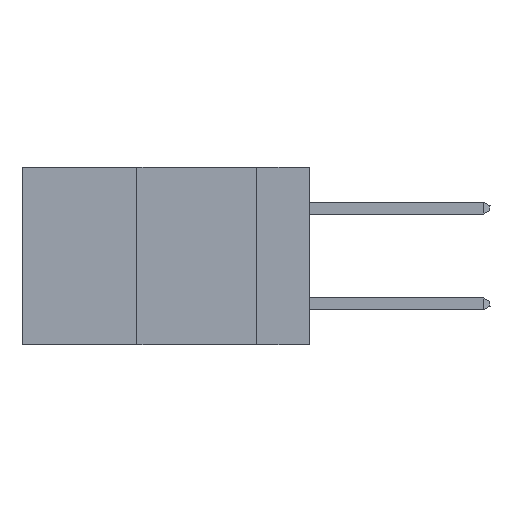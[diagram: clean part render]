
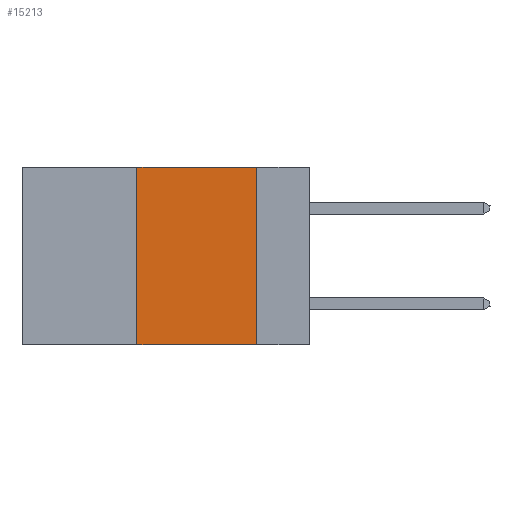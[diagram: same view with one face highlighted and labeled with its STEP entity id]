
A CAD part, left-side view. The second image highlights one B-rep face of the part: STEP entity #15213.
In plain terms, the highlighted planar face has unit normal (-1, 0, 0).
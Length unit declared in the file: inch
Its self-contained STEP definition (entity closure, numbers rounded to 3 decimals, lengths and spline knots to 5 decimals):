
#1571 = FACE_OUTER_BOUND ( 'NONE', #30304, .T. ) ;
#1800 = CARTESIAN_POINT ( 'NONE',  ( 0., 0.6, 0. ) ) ;
#1911 = DIRECTION ( 'NONE',  ( 1., 0., 0. ) ) ;
#2174 = VECTOR ( 'NONE', #3909, 39.37008 ) ;
#2556 = VECTOR ( 'NONE', #25964, 39.37008 ) ;
#3476 = EDGE_CURVE ( 'NONE', #14570, #18994, #7457, .T. ) ;
#3909 = DIRECTION ( 'NONE',  ( 0., 0., -1. ) ) ;
#4589 = EDGE_CURVE ( 'NONE', #14570, #4740, #16240, .T. ) ;
#4740 = VERTEX_POINT ( 'NONE', #10432 ) ;
#5135 = DIRECTION ( 'NONE',  ( 0., -1., 0. ) ) ;
#5413 = LINE ( 'NONE', #17313, #27243 ) ;
#5538 = VECTOR ( 'NONE', #17317, 39.37008 ) ;
#7457 = LINE ( 'NONE', #13384, #2556 ) ;
#9058 = VERTEX_POINT ( 'NONE', #29361 ) ;
#9211 = AXIS2_PLACEMENT_3D ( 'NONE', #1800, #1911, #11450 ) ;
#10432 = CARTESIAN_POINT ( 'NONE',  ( 0., 0.11, -0.37 ) ) ;
#11450 = DIRECTION ( 'NONE',  ( 0., 0., -1. ) ) ;
#13384 = CARTESIAN_POINT ( 'NONE',  ( 0., 0.36, 0. ) ) ;
#14570 = VERTEX_POINT ( 'NONE', #27188 ) ;
#15213 = ADVANCED_FACE ( 'NONE', ( #1571 ), #26151, .F. ) ;
#15814 = ORIENTED_EDGE ( 'NONE', *, *, #21680, .F. ) ;
#16240 = LINE ( 'NONE', #24626, #5538 ) ;
#17313 = CARTESIAN_POINT ( 'NONE',  ( 0., 0.6, 0. ) ) ;
#17317 = DIRECTION ( 'NONE',  ( 0., -1., 0. ) ) ;
#18544 = CARTESIAN_POINT ( 'NONE',  ( 0., 0.11, 0. ) ) ;
#18994 = VERTEX_POINT ( 'NONE', #26664 ) ;
#19139 = ORIENTED_EDGE ( 'NONE', *, *, #3476, .F. ) ;
#21283 = LINE ( 'NONE', #18544, #2174 ) ;
#21680 = EDGE_CURVE ( 'NONE', #9058, #4740, #21283, .T. ) ;
#24626 = CARTESIAN_POINT ( 'NONE',  ( 0., 0.6, -0.37 ) ) ;
#25964 = DIRECTION ( 'NONE',  ( 0., 0., 1. ) ) ;
#26151 = PLANE ( 'NONE',  #9211 ) ;
#26664 = CARTESIAN_POINT ( 'NONE',  ( 0., 0.36, 0. ) ) ;
#27188 = CARTESIAN_POINT ( 'NONE',  ( 0., 0.36, -0.37 ) ) ;
#27243 = VECTOR ( 'NONE', #5135, 39.37008 ) ;
#29361 = CARTESIAN_POINT ( 'NONE',  ( 0., 0.11, 0. ) ) ;
#30304 = EDGE_LOOP ( 'NONE', ( #15814, #30993, #19139, #30521 ) ) ;
#30521 = ORIENTED_EDGE ( 'NONE', *, *, #4589, .T. ) ;
#30713 = EDGE_CURVE ( 'NONE', #18994, #9058, #5413, .T. ) ;
#30993 = ORIENTED_EDGE ( 'NONE', *, *, #30713, .F. ) ;
